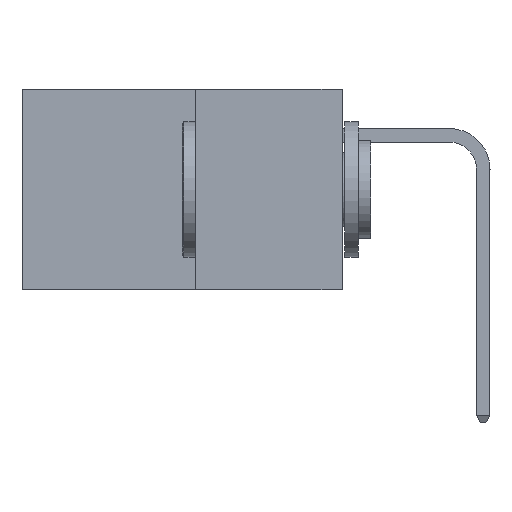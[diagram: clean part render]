
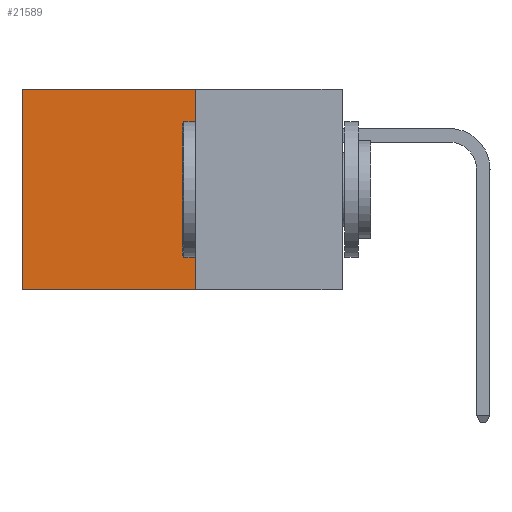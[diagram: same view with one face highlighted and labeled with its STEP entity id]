
A CAD part, left-side view. The second image highlights one B-rep face of the part: STEP entity #21589.
In plain terms, the highlighted planar face has unit normal (-1, 0, 0).
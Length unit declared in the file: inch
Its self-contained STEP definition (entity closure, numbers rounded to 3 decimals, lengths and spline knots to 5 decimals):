
#44 = AXIS2_PLACEMENT_3D ( 'NONE', #11948, #167, #13910 ) ;
#85 = PLANE ( 'NONE',  #44 ) ;
#167 = DIRECTION ( 'NONE',  ( 1., 0., 0. ) ) ;
#194 = ORIENTED_EDGE ( 'NONE', *, *, #4448, .F. ) ;
#2235 = CARTESIAN_POINT ( 'NONE',  ( 0.277, 0.27, -0.37 ) ) ;
#2796 = DIRECTION ( 'NONE',  ( 0., 1., 0. ) ) ;
#2985 = FACE_OUTER_BOUND ( 'NONE', #9977, .T. ) ;
#4448 = EDGE_CURVE ( 'NONE', #12629, #5810, #21138, .T. ) ;
#4532 = DIRECTION ( 'NONE',  ( 0., 1., 0. ) ) ;
#4710 = EDGE_CURVE ( 'NONE', #10696, #5810, #20217, .T. ) ;
#5009 = CARTESIAN_POINT ( 'NONE',  ( 0.277, 0.27, -0.37 ) ) ;
#5287 = LINE ( 'NONE', #10920, #10434 ) ;
#5810 = VERTEX_POINT ( 'NONE', #8959 ) ;
#7460 = EDGE_CURVE ( 'NONE', #13402, #10696, #19764, .T. ) ;
#8959 = CARTESIAN_POINT ( 'NONE',  ( 0.277, 0.59, -0.37 ) ) ;
#9977 = EDGE_LOOP ( 'NONE', ( #22068, #194, #12800, #21006 ) ) ;
#10434 = VECTOR ( 'NONE', #12891, 39.37008 ) ;
#10696 = VERTEX_POINT ( 'NONE', #12421 ) ;
#10920 = CARTESIAN_POINT ( 'NONE',  ( 0.277, 0.27, -0.37 ) ) ;
#11948 = CARTESIAN_POINT ( 'NONE',  ( 0.277, 0.27, -0.37 ) ) ;
#12421 = CARTESIAN_POINT ( 'NONE',  ( 0.277, 0.59, 0. ) ) ;
#12543 = CARTESIAN_POINT ( 'NONE',  ( 0.277, 0.27, 0. ) ) ;
#12629 = VERTEX_POINT ( 'NONE', #2235 ) ;
#12800 = ORIENTED_EDGE ( 'NONE', *, *, #12933, .F. ) ;
#12891 = DIRECTION ( 'NONE',  ( 0., 0., -1. ) ) ;
#12933 = EDGE_CURVE ( 'NONE', #13402, #12629, #5287, .T. ) ;
#13402 = VERTEX_POINT ( 'NONE', #14314 ) ;
#13910 = DIRECTION ( 'NONE',  ( 0., 0., -1. ) ) ;
#14314 = CARTESIAN_POINT ( 'NONE',  ( 0.277, 0.27, 0. ) ) ;
#15957 = VECTOR ( 'NONE', #4532, 39.37008 ) ;
#18415 = CARTESIAN_POINT ( 'NONE',  ( 0.277, 0.59, -0.37 ) ) ;
#18418 = DIRECTION ( 'NONE',  ( 0., 0., -1. ) ) ;
#19011 = VECTOR ( 'NONE', #18418, 39.37008 ) ;
#19157 = VECTOR ( 'NONE', #2796, 39.37008 ) ;
#19764 = LINE ( 'NONE', #12543, #19157 ) ;
#20217 = LINE ( 'NONE', #18415, #19011 ) ;
#21006 = ORIENTED_EDGE ( 'NONE', *, *, #7460, .T. ) ;
#21138 = LINE ( 'NONE', #5009, #15957 ) ;
#21589 = ADVANCED_FACE ( 'NONE', ( #2985 ), #85, .F. ) ;
#22068 = ORIENTED_EDGE ( 'NONE', *, *, #4710, .T. ) ;
